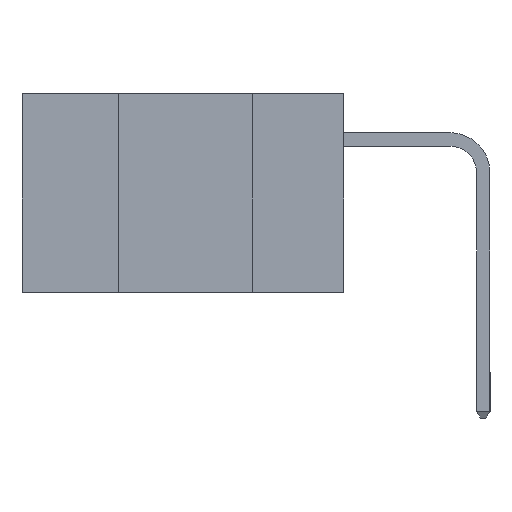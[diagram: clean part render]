
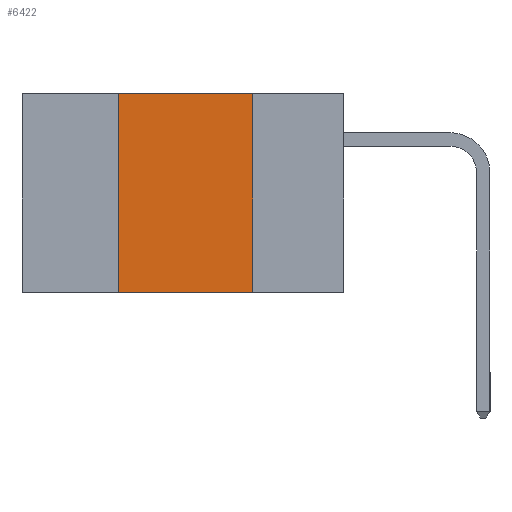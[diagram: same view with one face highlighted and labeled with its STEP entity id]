
A CAD part, left-side view. The second image highlights one B-rep face of the part: STEP entity #6422.
In plain terms, the highlighted planar face has unit normal (-1, 0, 0).
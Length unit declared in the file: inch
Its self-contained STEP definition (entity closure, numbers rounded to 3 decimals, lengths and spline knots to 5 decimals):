
#347 = VECTOR ( 'NONE', #11459, 39.37008 ) ;
#357 = DIRECTION ( 'NONE',  ( 0., -1., 0. ) ) ;
#424 = VERTEX_POINT ( 'NONE', #16688 ) ;
#1944 = EDGE_CURVE ( 'NONE', #17556, #2180, #6297, .T. ) ;
#2105 = VERTEX_POINT ( 'NONE', #16587 ) ;
#2180 = VERTEX_POINT ( 'NONE', #23994 ) ;
#2252 = CARTESIAN_POINT ( 'NONE',  ( 0., 0.6, 0. ) ) ;
#2907 = DIRECTION ( 'NONE',  ( 0., -1., 0. ) ) ;
#4107 = DIRECTION ( 'NONE',  ( 1., 0., 0. ) ) ;
#5023 = ORIENTED_EDGE ( 'NONE', *, *, #24296, .F. ) ;
#5644 = LINE ( 'NONE', #17175, #347 ) ;
#5815 = EDGE_LOOP ( 'NONE', ( #5023, #20902, #15041, #14593 ) ) ;
#6221 = CARTESIAN_POINT ( 'NONE',  ( 0., 0.17, -0.37 ) ) ;
#6297 = LINE ( 'NONE', #15256, #10413 ) ;
#6422 = ADVANCED_FACE ( 'NONE', ( #6456 ), #10294, .F. ) ;
#6456 = FACE_OUTER_BOUND ( 'NONE', #5815, .T. ) ;
#6910 = VECTOR ( 'NONE', #21456, 39.37008 ) ;
#7205 = EDGE_CURVE ( 'NONE', #2105, #17556, #5644, .T. ) ;
#7466 = AXIS2_PLACEMENT_3D ( 'NONE', #2252, #4107, #19599 ) ;
#10294 = PLANE ( 'NONE',  #7466 ) ;
#10413 = VECTOR ( 'NONE', #357, 39.37008 ) ;
#10695 = CARTESIAN_POINT ( 'NONE',  ( 0., 0.6, -0.37 ) ) ;
#11459 = DIRECTION ( 'NONE',  ( 0., 0., 1. ) ) ;
#11605 = EDGE_CURVE ( 'NONE', #2105, #424, #21849, .T. ) ;
#11927 = LINE ( 'NONE', #6221, #6910 ) ;
#14593 = ORIENTED_EDGE ( 'NONE', *, *, #11605, .T. ) ;
#15041 = ORIENTED_EDGE ( 'NONE', *, *, #7205, .F. ) ;
#15256 = CARTESIAN_POINT ( 'NONE',  ( 0., 0.6, 0. ) ) ;
#16587 = CARTESIAN_POINT ( 'NONE',  ( 0., 0.42, -0.37 ) ) ;
#16688 = CARTESIAN_POINT ( 'NONE',  ( 0., 0.17, -0.37 ) ) ;
#17104 = CARTESIAN_POINT ( 'NONE',  ( 0., 0.42, 0. ) ) ;
#17175 = CARTESIAN_POINT ( 'NONE',  ( 0., 0.42, -0.37 ) ) ;
#17556 = VERTEX_POINT ( 'NONE', #17104 ) ;
#19599 = DIRECTION ( 'NONE',  ( 0., 0., -1. ) ) ;
#20902 = ORIENTED_EDGE ( 'NONE', *, *, #1944, .F. ) ;
#20933 = VECTOR ( 'NONE', #2907, 39.37008 ) ;
#21456 = DIRECTION ( 'NONE',  ( 0., 0., -1. ) ) ;
#21849 = LINE ( 'NONE', #10695, #20933 ) ;
#23994 = CARTESIAN_POINT ( 'NONE',  ( 0., 0.17, 0. ) ) ;
#24296 = EDGE_CURVE ( 'NONE', #2180, #424, #11927, .T. ) ;
